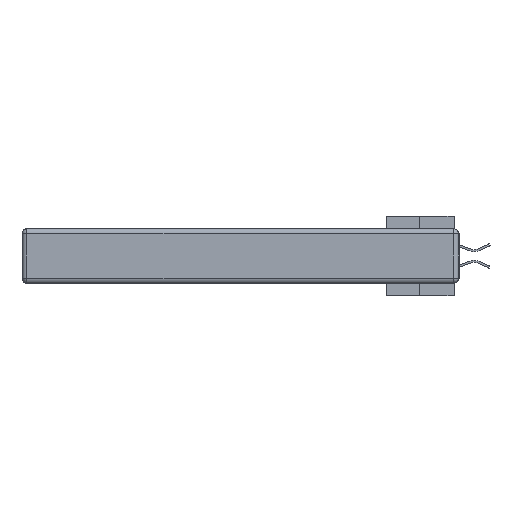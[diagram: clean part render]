
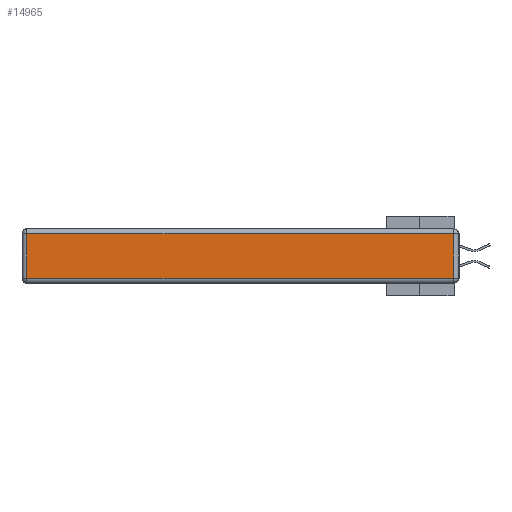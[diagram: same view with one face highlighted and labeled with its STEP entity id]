
A CAD part, left-side view. The second image highlights one B-rep face of the part: STEP entity #14965.
In plain terms, the highlighted planar face has unit normal (-1, 0, 0).
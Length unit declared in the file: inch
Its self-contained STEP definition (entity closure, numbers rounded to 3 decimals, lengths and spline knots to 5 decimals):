
#1301 = VECTOR ( 'NONE', #16975, 39.37008 ) ;
#4082 = ORIENTED_EDGE ( 'NONE', *, *, #22082, .T. ) ;
#4203 = VECTOR ( 'NONE', #9307, 39.37008 ) ;
#6418 = PLANE ( 'NONE',  #26483 ) ;
#6613 = CARTESIAN_POINT ( 'NONE',  ( 0., 0.03, -0.343 ) ) ;
#7631 = EDGE_CURVE ( 'NONE', #21344, #35456, #13655, .T. ) ;
#9307 = DIRECTION ( 'NONE',  ( 0., 0., 1. ) ) ;
#10149 = VECTOR ( 'NONE', #15848, 39.37008 ) ;
#10576 = CARTESIAN_POINT ( 'NONE',  ( 0., 2.72, -0.313 ) ) ;
#11049 = EDGE_CURVE ( 'NONE', #34140, #21344, #14648, .T. ) ;
#13413 = CARTESIAN_POINT ( 'NONE',  ( 0., 0.03, -0.03 ) ) ;
#13655 = LINE ( 'NONE', #15627, #10149 ) ;
#14029 = LINE ( 'NONE', #25783, #24018 ) ;
#14648 = LINE ( 'NONE', #6613, #4203 ) ;
#14965 = ADVANCED_FACE ( 'NONE', ( #21200 ), #6418, .T. ) ;
#15627 = CARTESIAN_POINT ( 'NONE',  ( 0., 2.75, -0.03 ) ) ;
#15848 = DIRECTION ( 'NONE',  ( 0., 1., 0. ) ) ;
#16627 = ORIENTED_EDGE ( 'NONE', *, *, #11049, .T. ) ;
#16856 = CARTESIAN_POINT ( 'NONE',  ( 0., 0., -0.313 ) ) ;
#16975 = DIRECTION ( 'NONE',  ( 0., -1., 0. ) ) ;
#17665 = EDGE_LOOP ( 'NONE', ( #22265, #16627, #22336, #4082 ) ) ;
#18805 = CARTESIAN_POINT ( 'NONE',  ( 0., 0.03, -0.313 ) ) ;
#21200 = FACE_OUTER_BOUND ( 'NONE', #17665, .T. ) ;
#21344 = VERTEX_POINT ( 'NONE', #13413 ) ;
#22082 = EDGE_CURVE ( 'NONE', #35456, #28822, #14029, .T. ) ;
#22265 = ORIENTED_EDGE ( 'NONE', *, *, #35474, .T. ) ;
#22336 = ORIENTED_EDGE ( 'NONE', *, *, #7631, .T. ) ;
#24018 = VECTOR ( 'NONE', #31401, 39.37008 ) ;
#25343 = CARTESIAN_POINT ( 'NONE',  ( 0., 2.72, -0.03 ) ) ;
#25783 = CARTESIAN_POINT ( 'NONE',  ( 0., 2.72, -0.343 ) ) ;
#26483 = AXIS2_PLACEMENT_3D ( 'NONE', #31583, #34449, #28389 ) ;
#28250 = LINE ( 'NONE', #16856, #1301 ) ;
#28389 = DIRECTION ( 'NONE',  ( 0., 0., 1. ) ) ;
#28822 = VERTEX_POINT ( 'NONE', #10576 ) ;
#31401 = DIRECTION ( 'NONE',  ( 0., 0., -1. ) ) ;
#31583 = CARTESIAN_POINT ( 'NONE',  ( 0., 0., -0.343 ) ) ;
#34140 = VERTEX_POINT ( 'NONE', #18805 ) ;
#34449 = DIRECTION ( 'NONE',  ( -1., 0., 0. ) ) ;
#35456 = VERTEX_POINT ( 'NONE', #25343 ) ;
#35474 = EDGE_CURVE ( 'NONE', #28822, #34140, #28250, .T. ) ;
